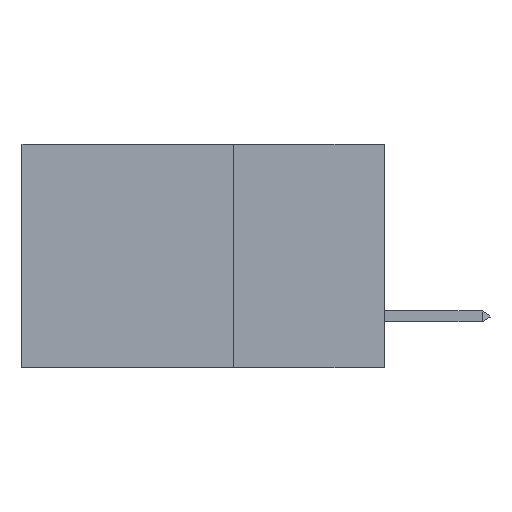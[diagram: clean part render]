
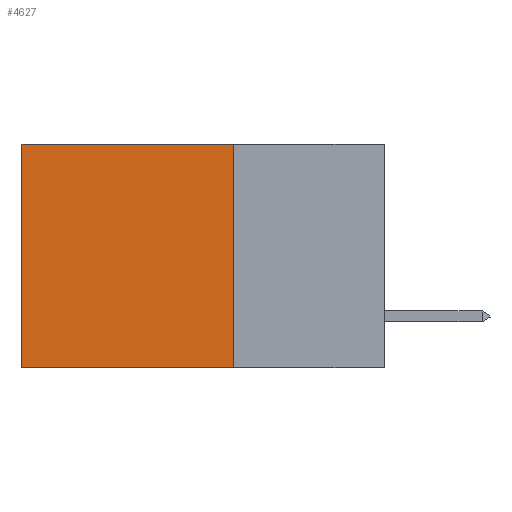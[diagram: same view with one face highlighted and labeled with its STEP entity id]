
A CAD part, left-side view. The second image highlights one B-rep face of the part: STEP entity #4627.
In plain terms, the highlighted planar face has unit normal (-1, 0, 0).
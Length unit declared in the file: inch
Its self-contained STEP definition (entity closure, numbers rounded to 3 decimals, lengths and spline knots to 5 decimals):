
#539 = VERTEX_POINT ( 'NONE', #13344 ) ;
#831 = LINE ( 'NONE', #10530, #7601 ) ;
#910 = DIRECTION ( 'NONE',  ( 0., 0., -1. ) ) ;
#1898 = CARTESIAN_POINT ( 'NONE',  ( 0.2875, 0.25, 0. ) ) ;
#1909 = CARTESIAN_POINT ( 'NONE',  ( 0.2875, 0.6, -0.37 ) ) ;
#1972 = PLANE ( 'NONE',  #9828 ) ;
#1998 = VERTEX_POINT ( 'NONE', #8017 ) ;
#2125 = EDGE_CURVE ( 'NONE', #4260, #1998, #9649, .T. ) ;
#2729 = EDGE_CURVE ( 'NONE', #1998, #8989, #831, .T. ) ;
#3231 = ORIENTED_EDGE ( 'NONE', *, *, #5464, .T. ) ;
#4186 = VECTOR ( 'NONE', #12568, 39.37008 ) ;
#4260 = VERTEX_POINT ( 'NONE', #11256 ) ;
#4627 = ADVANCED_FACE ( 'NONE', ( #4788 ), #1972, .F. ) ;
#4788 = FACE_OUTER_BOUND ( 'NONE', #5783, .T. ) ;
#5309 = VECTOR ( 'NONE', #910, 39.37008 ) ;
#5464 = EDGE_CURVE ( 'NONE', #4260, #539, #10499, .T. ) ;
#5783 = EDGE_LOOP ( 'NONE', ( #12101, #6117, #13298, #3231 ) ) ;
#6117 = ORIENTED_EDGE ( 'NONE', *, *, #2729, .F. ) ;
#6519 = CARTESIAN_POINT ( 'NONE',  ( 0.2875, 0.6, 0. ) ) ;
#7601 = VECTOR ( 'NONE', #13728, 39.37008 ) ;
#8017 = CARTESIAN_POINT ( 'NONE',  ( 0.2875, 0.25, -0.37 ) ) ;
#8815 = VECTOR ( 'NONE', #12227, 39.37008 ) ;
#8989 = VERTEX_POINT ( 'NONE', #1909 ) ;
#9649 = LINE ( 'NONE', #11098, #8815 ) ;
#9762 = DIRECTION ( 'NONE',  ( 1., 0., 0. ) ) ;
#9828 = AXIS2_PLACEMENT_3D ( 'NONE', #11823, #9762, #13059 ) ;
#10476 = LINE ( 'NONE', #6519, #5309 ) ;
#10499 = LINE ( 'NONE', #1898, #4186 ) ;
#10530 = CARTESIAN_POINT ( 'NONE',  ( 0.2875, 0.25, -0.37 ) ) ;
#11098 = CARTESIAN_POINT ( 'NONE',  ( 0.2875, 0.25, 0. ) ) ;
#11256 = CARTESIAN_POINT ( 'NONE',  ( 0.2875, 0.25, 0. ) ) ;
#11823 = CARTESIAN_POINT ( 'NONE',  ( 0.2875, 0.25, 0. ) ) ;
#12101 = ORIENTED_EDGE ( 'NONE', *, *, #12877, .T. ) ;
#12227 = DIRECTION ( 'NONE',  ( 0., 0., -1. ) ) ;
#12568 = DIRECTION ( 'NONE',  ( 0., 1., 0. ) ) ;
#12877 = EDGE_CURVE ( 'NONE', #539, #8989, #10476, .T. ) ;
#13059 = DIRECTION ( 'NONE',  ( 0., 0., -1. ) ) ;
#13298 = ORIENTED_EDGE ( 'NONE', *, *, #2125, .F. ) ;
#13344 = CARTESIAN_POINT ( 'NONE',  ( 0.2875, 0.6, 0. ) ) ;
#13728 = DIRECTION ( 'NONE',  ( 0., 1., 0. ) ) ;
